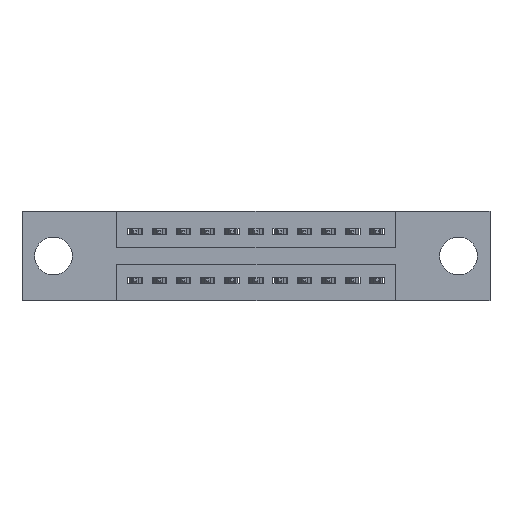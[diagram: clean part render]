
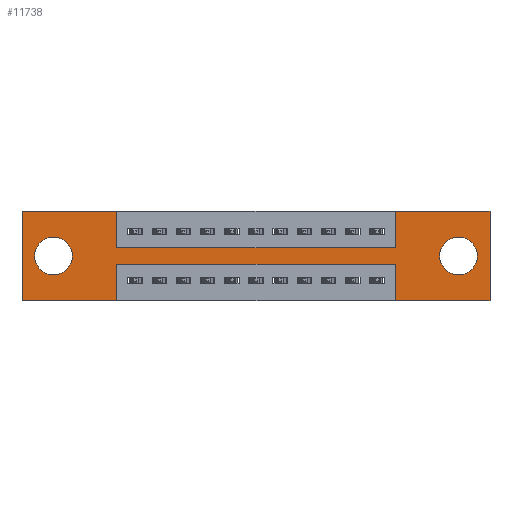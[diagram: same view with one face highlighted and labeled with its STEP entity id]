
A CAD part, front view. The second image highlights one B-rep face of the part: STEP entity #11738.
In plain terms, the highlighted planar face has unit normal (0, -1, 0).
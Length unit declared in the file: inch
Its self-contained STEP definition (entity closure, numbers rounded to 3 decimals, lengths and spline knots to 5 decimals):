
#51 = AXIS2_PLACEMENT_3D ( 'NONE', #11179, #8396, #9375 ) ;
#81 = DIRECTION ( 'NONE',  ( -1., 0., 0. ) ) ;
#235 = ORIENTED_EDGE ( 'NONE', *, *, #8049, .T. ) ;
#268 = VERTEX_POINT ( 'NONE', #9582 ) ;
#609 = CARTESIAN_POINT ( 'NONE',  ( 0.3925, 0., -0.37 ) ) ;
#644 = CARTESIAN_POINT ( 'NONE',  ( 0., 0., 0. ) ) ;
#747 = VECTOR ( 'NONE', #4600, 39.37008 ) ;
#807 = CARTESIAN_POINT ( 'NONE',  ( 1.805, 0., -0.107 ) ) ;
#818 = ORIENTED_EDGE ( 'NONE', *, *, #6728, .F. ) ;
#911 = LINE ( 'NONE', #3591, #6317 ) ;
#1134 = ORIENTED_EDGE ( 'NONE', *, *, #12390, .T. ) ;
#1227 = DIRECTION ( 'NONE',  ( 1., 0., 0. ) ) ;
#1238 = CARTESIAN_POINT ( 'NONE',  ( 1.805, 0., -0.263 ) ) ;
#1287 = CARTESIAN_POINT ( 'NONE',  ( 1.5425, 0., 0. ) ) ;
#1434 = EDGE_CURVE ( 'NONE', #10264, #2424, #10494, .T. ) ;
#1543 = EDGE_CURVE ( 'NONE', #2213, #6591, #911, .T. ) ;
#1557 = EDGE_CURVE ( 'NONE', #10716, #2213, #3381, .T. ) ;
#1621 = VECTOR ( 'NONE', #12347, 39.37008 ) ;
#1622 = EDGE_CURVE ( 'NONE', #6682, #10812, #6607, .T. ) ;
#1665 = DIRECTION ( 'NONE',  ( 0., 1., 0. ) ) ;
#1673 = VECTOR ( 'NONE', #1227, 39.37008 ) ;
#1740 = AXIS2_PLACEMENT_3D ( 'NONE', #8841, #5901, #3923 ) ;
#1771 = CARTESIAN_POINT ( 'NONE',  ( 1.5425, 0., -0.37 ) ) ;
#1826 = DIRECTION ( 'NONE',  ( -1., 0., 0. ) ) ;
#1930 = LINE ( 'NONE', #2457, #1621 ) ;
#2014 = DIRECTION ( 'NONE',  ( 0., 0., 1. ) ) ;
#2100 = DIRECTION ( 'NONE',  ( -1., 0., 0. ) ) ;
#2213 = VERTEX_POINT ( 'NONE', #2691 ) ;
#2242 = ORIENTED_EDGE ( 'NONE', *, *, #2320, .F. ) ;
#2320 = EDGE_CURVE ( 'NONE', #3031, #5102, #5680, .T. ) ;
#2424 = VERTEX_POINT ( 'NONE', #3401 ) ;
#2445 = CARTESIAN_POINT ( 'NONE',  ( 1.935, 0., 0. ) ) ;
#2451 = VECTOR ( 'NONE', #81, 39.37008 ) ;
#2457 = CARTESIAN_POINT ( 'NONE',  ( 0.3925, 0., -0.15 ) ) ;
#2470 = CARTESIAN_POINT ( 'NONE',  ( 1.5425, 0., -0.22 ) ) ;
#2553 = EDGE_LOOP ( 'NONE', ( #235, #9833 ) ) ;
#2691 = CARTESIAN_POINT ( 'NONE',  ( 1.935, 0., -0.37 ) ) ;
#2897 = LINE ( 'NONE', #5106, #2451 ) ;
#2989 = DIRECTION ( 'NONE',  ( 0., 0., 1. ) ) ;
#3031 = VERTEX_POINT ( 'NONE', #9842 ) ;
#3046 = VECTOR ( 'NONE', #11775, 39.37008 ) ;
#3069 = ORIENTED_EDGE ( 'NONE', *, *, #1543, .F. ) ;
#3092 = CARTESIAN_POINT ( 'NONE',  ( 0.13, 0., -0.185 ) ) ;
#3167 = CARTESIAN_POINT ( 'NONE',  ( 0., 0., 0. ) ) ;
#3218 = VECTOR ( 'NONE', #7968, 39.37008 ) ;
#3294 = ORIENTED_EDGE ( 'NONE', *, *, #8592, .T. ) ;
#3306 = LINE ( 'NONE', #3915, #4688 ) ;
#3381 = LINE ( 'NONE', #2445, #747 ) ;
#3401 = CARTESIAN_POINT ( 'NONE',  ( 0.3925, 0., -0.22 ) ) ;
#3591 = CARTESIAN_POINT ( 'NONE',  ( 0., 0., -0.37 ) ) ;
#3753 = CARTESIAN_POINT ( 'NONE',  ( 0., 0., 0. ) ) ;
#3775 = PLANE ( 'NONE',  #51 ) ;
#3790 = ORIENTED_EDGE ( 'NONE', *, *, #1557, .F. ) ;
#3915 = CARTESIAN_POINT ( 'NONE',  ( 0.3925, 0., 0. ) ) ;
#3923 = DIRECTION ( 'NONE',  ( 0., 0., 1. ) ) ;
#4013 = VERTEX_POINT ( 'NONE', #12215 ) ;
#4319 = LINE ( 'NONE', #3167, #1673 ) ;
#4348 = EDGE_LOOP ( 'NONE', ( #10214, #9354, #12425, #3069, #3790, #8373, #2242, #5041, #10395, #818, #5635, #11260 ) ) ;
#4359 = VERTEX_POINT ( 'NONE', #807 ) ;
#4574 = CARTESIAN_POINT ( 'NONE',  ( 1.805, 0., -0.185 ) ) ;
#4600 = DIRECTION ( 'NONE',  ( 0., 0., -1. ) ) ;
#4625 = CARTESIAN_POINT ( 'NONE',  ( 0., 0., 0. ) ) ;
#4688 = VECTOR ( 'NONE', #5994, 39.37008 ) ;
#4866 = CARTESIAN_POINT ( 'NONE',  ( 1.5425, 0., 0. ) ) ;
#5041 = ORIENTED_EDGE ( 'NONE', *, *, #8866, .F. ) ;
#5102 = VERTEX_POINT ( 'NONE', #1287 ) ;
#5106 = CARTESIAN_POINT ( 'NONE',  ( 0., 0., -0.37 ) ) ;
#5635 = ORIENTED_EDGE ( 'NONE', *, *, #6532, .F. ) ;
#5680 = LINE ( 'NONE', #4866, #3046 ) ;
#5784 = LINE ( 'NONE', #7917, #11539 ) ;
#5901 = DIRECTION ( 'NONE',  ( 0., 1., 0. ) ) ;
#5994 = DIRECTION ( 'NONE',  ( 0., 0., -1. ) ) ;
#6317 = VECTOR ( 'NONE', #1826, 39.37008 ) ;
#6532 = EDGE_CURVE ( 'NONE', #4013, #6642, #8470, .T. ) ;
#6591 = VERTEX_POINT ( 'NONE', #1771 ) ;
#6607 = CIRCLE ( 'NONE', #1740, 0.078 ) ;
#6642 = VERTEX_POINT ( 'NONE', #3753 ) ;
#6682 = VERTEX_POINT ( 'NONE', #10707 ) ;
#6703 = DIRECTION ( 'NONE',  ( 0., 1., 0. ) ) ;
#6728 = EDGE_CURVE ( 'NONE', #6642, #10059, #4319, .T. ) ;
#6891 = CIRCLE ( 'NONE', #11982, 0.078 ) ;
#6956 = EDGE_CURVE ( 'NONE', #12584, #4013, #2897, .T. ) ;
#6982 = DIRECTION ( 'NONE',  ( 0., 1., 0. ) ) ;
#6992 = EDGE_CURVE ( 'NONE', #2424, #12584, #11144, .T. ) ;
#7020 = CARTESIAN_POINT ( 'NONE',  ( 0.3925, 0., -0.22 ) ) ;
#7582 = EDGE_LOOP ( 'NONE', ( #1134, #3294 ) ) ;
#7917 = CARTESIAN_POINT ( 'NONE',  ( 1.5425, 0., -0.37 ) ) ;
#7968 = DIRECTION ( 'NONE',  ( 0., 0., -1. ) ) ;
#7993 = AXIS2_PLACEMENT_3D ( 'NONE', #11646, #6703, #11733 ) ;
#8049 = EDGE_CURVE ( 'NONE', #10812, #6682, #6891, .T. ) ;
#8373 = ORIENTED_EDGE ( 'NONE', *, *, #10284, .F. ) ;
#8396 = DIRECTION ( 'NONE',  ( 0., -1., 0. ) ) ;
#8470 = LINE ( 'NONE', #4625, #12531 ) ;
#8592 = EDGE_CURVE ( 'NONE', #10033, #4359, #10596, .T. ) ;
#8801 = CIRCLE ( 'NONE', #7993, 0.078 ) ;
#8827 = FACE_BOUND ( 'NONE', #2553, .T. ) ;
#8841 = CARTESIAN_POINT ( 'NONE',  ( 0.13, 0., -0.185 ) ) ;
#8866 = EDGE_CURVE ( 'NONE', #268, #3031, #1930, .T. ) ;
#9124 = EDGE_CURVE ( 'NONE', #6591, #10264, #5784, .T. ) ;
#9183 = CARTESIAN_POINT ( 'NONE',  ( 1.935, 0., 0. ) ) ;
#9354 = ORIENTED_EDGE ( 'NONE', *, *, #1434, .F. ) ;
#9375 = DIRECTION ( 'NONE',  ( 0., 0., -1. ) ) ;
#9572 = FACE_BOUND ( 'NONE', #7582, .T. ) ;
#9582 = CARTESIAN_POINT ( 'NONE',  ( 0.3925, 0., -0.15 ) ) ;
#9783 = AXIS2_PLACEMENT_3D ( 'NONE', #4574, #1665, #10676 ) ;
#9833 = ORIENTED_EDGE ( 'NONE', *, *, #1622, .T. ) ;
#9842 = CARTESIAN_POINT ( 'NONE',  ( 1.5425, 0., -0.15 ) ) ;
#10033 = VERTEX_POINT ( 'NONE', #1238 ) ;
#10059 = VERTEX_POINT ( 'NONE', #12076 ) ;
#10214 = ORIENTED_EDGE ( 'NONE', *, *, #6992, .F. ) ;
#10264 = VERTEX_POINT ( 'NONE', #2470 ) ;
#10284 = EDGE_CURVE ( 'NONE', #5102, #10716, #11313, .T. ) ;
#10395 = ORIENTED_EDGE ( 'NONE', *, *, #10508, .F. ) ;
#10440 = CARTESIAN_POINT ( 'NONE',  ( 0.3925, 0., -0.37 ) ) ;
#10494 = LINE ( 'NONE', #7020, #11451 ) ;
#10495 = DIRECTION ( 'NONE',  ( 1., 0., 0. ) ) ;
#10508 = EDGE_CURVE ( 'NONE', #10059, #268, #3306, .T. ) ;
#10596 = CIRCLE ( 'NONE', #9783, 0.078 ) ;
#10619 = CARTESIAN_POINT ( 'NONE',  ( 0.13, 0., -0.107 ) ) ;
#10676 = DIRECTION ( 'NONE',  ( 0., 0., -1. ) ) ;
#10707 = CARTESIAN_POINT ( 'NONE',  ( 0.13, 0., -0.263 ) ) ;
#10716 = VERTEX_POINT ( 'NONE', #9183 ) ;
#10743 = DIRECTION ( 'NONE',  ( 0., 0., 1. ) ) ;
#10812 = VERTEX_POINT ( 'NONE', #10619 ) ;
#10839 = VECTOR ( 'NONE', #10495, 39.37008 ) ;
#11144 = LINE ( 'NONE', #10440, #3218 ) ;
#11179 = CARTESIAN_POINT ( 'NONE',  ( 0., 0., -0.37 ) ) ;
#11260 = ORIENTED_EDGE ( 'NONE', *, *, #6956, .F. ) ;
#11313 = LINE ( 'NONE', #644, #10839 ) ;
#11451 = VECTOR ( 'NONE', #2100, 39.37008 ) ;
#11539 = VECTOR ( 'NONE', #2989, 39.37008 ) ;
#11646 = CARTESIAN_POINT ( 'NONE',  ( 1.805, 0., -0.185 ) ) ;
#11733 = DIRECTION ( 'NONE',  ( 0., 0., -1. ) ) ;
#11738 = ADVANCED_FACE ( 'NONE', ( #9572, #8827, #11813 ), #3775, .T. ) ;
#11775 = DIRECTION ( 'NONE',  ( 0., 0., 1. ) ) ;
#11813 = FACE_OUTER_BOUND ( 'NONE', #4348, .T. ) ;
#11982 = AXIS2_PLACEMENT_3D ( 'NONE', #3092, #6982, #2014 ) ;
#12076 = CARTESIAN_POINT ( 'NONE',  ( 0.3925, 0., 0. ) ) ;
#12215 = CARTESIAN_POINT ( 'NONE',  ( 0., 0., -0.37 ) ) ;
#12347 = DIRECTION ( 'NONE',  ( 1., 0., 0. ) ) ;
#12390 = EDGE_CURVE ( 'NONE', #4359, #10033, #8801, .T. ) ;
#12425 = ORIENTED_EDGE ( 'NONE', *, *, #9124, .F. ) ;
#12531 = VECTOR ( 'NONE', #10743, 39.37008 ) ;
#12584 = VERTEX_POINT ( 'NONE', #609 ) ;
